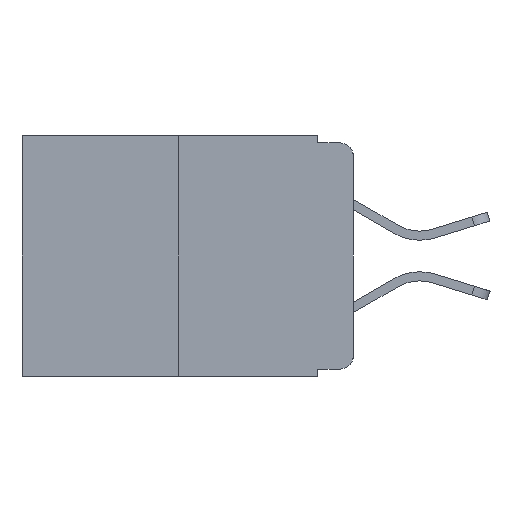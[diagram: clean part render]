
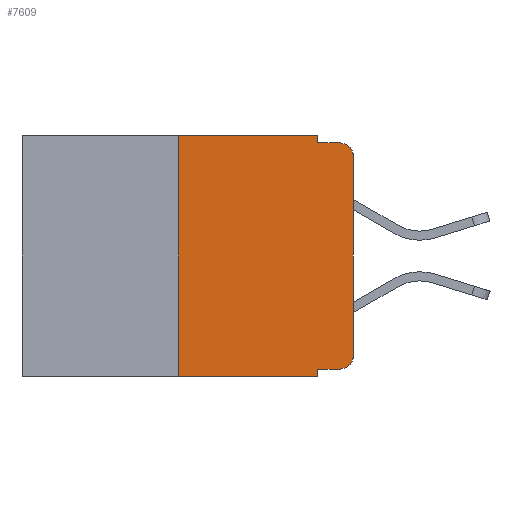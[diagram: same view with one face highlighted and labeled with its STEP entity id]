
A CAD part, left-side view. The second image highlights one B-rep face of the part: STEP entity #7609.
In plain terms, the highlighted planar face has unit normal (-1, 0, 0).
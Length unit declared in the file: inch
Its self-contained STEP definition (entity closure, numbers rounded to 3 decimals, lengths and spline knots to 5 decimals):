
#83 = CARTESIAN_POINT ( 'NONE',  ( 0., 0., 0. ) ) ;
#184 = CARTESIAN_POINT ( 'NONE',  ( 0., 0.051, -0.333 ) ) ;
#316 = CARTESIAN_POINT ( 'NONE',  ( 0., 0.02, -0.01 ) ) ;
#498 = LINE ( 'NONE', #11299, #13824 ) ;
#523 = LINE ( 'NONE', #13962, #10004 ) ;
#538 = VECTOR ( 'NONE', #6500, 39.37008 ) ;
#658 = CARTESIAN_POINT ( 'NONE',  ( 0., 0.473, 0. ) ) ;
#1022 = VERTEX_POINT ( 'NONE', #9566 ) ;
#1129 = EDGE_CURVE ( 'NONE', #13249, #9833, #6811, .T. ) ;
#1373 = ORIENTED_EDGE ( 'NONE', *, *, #5684, .T. ) ;
#1424 = ORIENTED_EDGE ( 'NONE', *, *, #11009, .F. ) ;
#1605 = LINE ( 'NONE', #14638, #538 ) ;
#1655 = ORIENTED_EDGE ( 'NONE', *, *, #14794, .F. ) ;
#2005 = LINE ( 'NONE', #4009, #2864 ) ;
#2049 = DIRECTION ( 'NONE',  ( -1., 0., 0. ) ) ;
#2215 = CARTESIAN_POINT ( 'NONE',  ( 0., 0.051, -0.343 ) ) ;
#2679 = ORIENTED_EDGE ( 'NONE', *, *, #2750, .F. ) ;
#2750 = EDGE_CURVE ( 'NONE', #13616, #8458, #498, .T. ) ;
#2864 = VECTOR ( 'NONE', #9667, 39.37008 ) ;
#3401 = VECTOR ( 'NONE', #3423, 39.37008 ) ;
#3423 = DIRECTION ( 'NONE',  ( 0., 0., 1. ) ) ;
#3588 = LINE ( 'NONE', #83, #3401 ) ;
#3589 = LINE ( 'NONE', #8605, #8244 ) ;
#4009 = CARTESIAN_POINT ( 'NONE',  ( 0., 0.051, -0.333 ) ) ;
#4160 = AXIS2_PLACEMENT_3D ( 'NONE', #14597, #2049, #10003 ) ;
#4671 = ORIENTED_EDGE ( 'NONE', *, *, #13658, .T. ) ;
#4770 = CIRCLE ( 'NONE', #4160, 0.02 ) ;
#5049 = ORIENTED_EDGE ( 'NONE', *, *, #8640, .T. ) ;
#5142 = CARTESIAN_POINT ( 'NONE',  ( 0., 0.051, 0. ) ) ;
#5217 = ORIENTED_EDGE ( 'NONE', *, *, #8167, .F. ) ;
#5269 = DIRECTION ( 'NONE',  ( 0., 0., -1. ) ) ;
#5521 = LINE ( 'NONE', #9674, #7833 ) ;
#5684 = EDGE_CURVE ( 'NONE', #1022, #5877, #4770, .T. ) ;
#5877 = VERTEX_POINT ( 'NONE', #9249 ) ;
#6393 = DIRECTION ( 'NONE',  ( 1., 0., 0. ) ) ;
#6500 = DIRECTION ( 'NONE',  ( 0., -1., 0. ) ) ;
#6544 = DIRECTION ( 'NONE',  ( 0., 0., 1. ) ) ;
#6764 = VERTEX_POINT ( 'NONE', #12479 ) ;
#6811 = CIRCLE ( 'NONE', #7099, 0.02 ) ;
#6916 = CARTESIAN_POINT ( 'NONE',  ( 0., 0., -0.03 ) ) ;
#7032 = DIRECTION ( 'NONE',  ( 0., -1., 0. ) ) ;
#7099 = AXIS2_PLACEMENT_3D ( 'NONE', #7608, #9857, #12112 ) ;
#7216 = FACE_OUTER_BOUND ( 'NONE', #9074, .T. ) ;
#7608 = CARTESIAN_POINT ( 'NONE',  ( 0., 0.02, -0.03 ) ) ;
#7609 = ADVANCED_FACE ( 'NONE', ( #7216 ), #14436, .F. ) ;
#7742 = DIRECTION ( 'NONE',  ( 0., 0., -1. ) ) ;
#7833 = VECTOR ( 'NONE', #5269, 39.37008 ) ;
#8167 = EDGE_CURVE ( 'NONE', #8499, #12322, #13186, .T. ) ;
#8244 = VECTOR ( 'NONE', #12296, 39.37008 ) ;
#8458 = VERTEX_POINT ( 'NONE', #10346 ) ;
#8499 = VERTEX_POINT ( 'NONE', #184 ) ;
#8605 = CARTESIAN_POINT ( 'NONE',  ( 0., 0.473, 0. ) ) ;
#8640 = EDGE_CURVE ( 'NONE', #8499, #1022, #2005, .T. ) ;
#8786 = ORIENTED_EDGE ( 'NONE', *, *, #13229, .T. ) ;
#8891 = CARTESIAN_POINT ( 'NONE',  ( 0., 0.25, -0.343 ) ) ;
#9074 = EDGE_LOOP ( 'NONE', ( #8786, #13365, #14209, #1655, #1424, #2679, #4671, #5217, #5049, #1373 ) ) ;
#9249 = CARTESIAN_POINT ( 'NONE',  ( 0., 0., -0.313 ) ) ;
#9566 = CARTESIAN_POINT ( 'NONE',  ( 0., 0.02, -0.333 ) ) ;
#9667 = DIRECTION ( 'NONE',  ( 0., -1., 0. ) ) ;
#9674 = CARTESIAN_POINT ( 'NONE',  ( 0., 0.051, 0. ) ) ;
#9827 = CARTESIAN_POINT ( 'NONE',  ( 0., 0.051, 0. ) ) ;
#9833 = VERTEX_POINT ( 'NONE', #316 ) ;
#9857 = DIRECTION ( 'NONE',  ( -1., 0., 0. ) ) ;
#10003 = DIRECTION ( 'NONE',  ( 0., 0., -1. ) ) ;
#10004 = VECTOR ( 'NONE', #7032, 39.37008 ) ;
#10346 = CARTESIAN_POINT ( 'NONE',  ( 0., 0.25, 0. ) ) ;
#11009 = EDGE_CURVE ( 'NONE', #8458, #13494, #3589, .T. ) ;
#11299 = CARTESIAN_POINT ( 'NONE',  ( 0., 0.25, 0. ) ) ;
#11575 = VECTOR ( 'NONE', #7742, 39.37008 ) ;
#12112 = DIRECTION ( 'NONE',  ( 0., 0., -1. ) ) ;
#12296 = DIRECTION ( 'NONE',  ( 0., -1., 0. ) ) ;
#12322 = VERTEX_POINT ( 'NONE', #2215 ) ;
#12479 = CARTESIAN_POINT ( 'NONE',  ( 0., 0.051, -0.01 ) ) ;
#13186 = LINE ( 'NONE', #9827, #11575 ) ;
#13229 = EDGE_CURVE ( 'NONE', #5877, #13249, #3588, .T. ) ;
#13249 = VERTEX_POINT ( 'NONE', #6916 ) ;
#13264 = AXIS2_PLACEMENT_3D ( 'NONE', #658, #6393, #13334 ) ;
#13334 = DIRECTION ( 'NONE',  ( 0., 0., -1. ) ) ;
#13365 = ORIENTED_EDGE ( 'NONE', *, *, #1129, .T. ) ;
#13494 = VERTEX_POINT ( 'NONE', #5142 ) ;
#13616 = VERTEX_POINT ( 'NONE', #8891 ) ;
#13658 = EDGE_CURVE ( 'NONE', #13616, #12322, #1605, .T. ) ;
#13824 = VECTOR ( 'NONE', #6544, 39.37008 ) ;
#13948 = EDGE_CURVE ( 'NONE', #6764, #9833, #523, .T. ) ;
#13962 = CARTESIAN_POINT ( 'NONE',  ( 0., 0.051, -0.01 ) ) ;
#14209 = ORIENTED_EDGE ( 'NONE', *, *, #13948, .F. ) ;
#14436 = PLANE ( 'NONE',  #13264 ) ;
#14597 = CARTESIAN_POINT ( 'NONE',  ( 0., 0.02, -0.313 ) ) ;
#14638 = CARTESIAN_POINT ( 'NONE',  ( 0., 0.473, -0.343 ) ) ;
#14794 = EDGE_CURVE ( 'NONE', #13494, #6764, #5521, .T. ) ;
